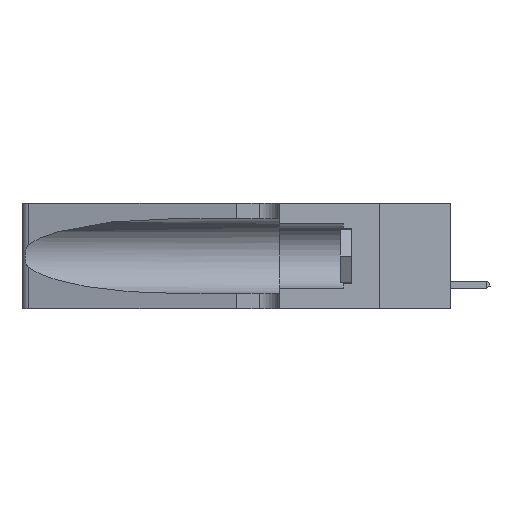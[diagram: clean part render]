
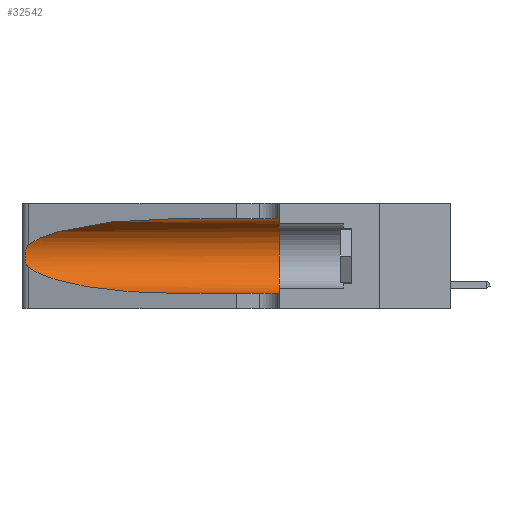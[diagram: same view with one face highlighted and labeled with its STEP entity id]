
A CAD part, left-side view. The second image highlights one B-rep face of the part: STEP entity #32542.
In plain terms, the highlighted cylindrical face has radius 3.308 mm (diameter 6.617 mm), a partial arc.
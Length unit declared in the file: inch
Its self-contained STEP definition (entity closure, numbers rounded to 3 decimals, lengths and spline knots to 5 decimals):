
#226 = CARTESIAN_POINT ( 'NONE',  ( 0.25487, 1.22718, 0.22369 ) ) ;
#278 = CIRCLE ( 'NONE', #18282, 0.13025 ) ;
#740 = ORIENTED_EDGE ( 'NONE', *, *, #19735, .T. ) ;
#765 = VERTEX_POINT ( 'NONE', #9057 ) ;
#1248 = CARTESIAN_POINT ( 'NONE',  ( 0.1305, 1.61858, 0.05475 ) ) ;
#1630 = CARTESIAN_POINT ( 'NONE',  ( 0.1305, 0.35, 0.05475 ) ) ;
#2726 = CARTESIAN_POINT ( 'NONE',  ( 0.26075, 1.23896, 0.178 ) ) ;
#3326 = CARTESIAN_POINT ( 'NONE',  ( 0.1305, 1.61858, 0.31525 ) ) ;
#3805 = ORIENTED_EDGE ( 'NONE', *, *, #20545, .T. ) ;
#3929 = B_SPLINE_CURVE_WITH_KNOTS ( 'NONE', 3,
 ( #226, #7706, #4819, #17422, #25188, #22457, #17846, #2726, #7383, #14912, #22665, #12674, #10114, #32436 ),
 .UNSPECIFIED., .F., .F.,
 ( 4, 2, 2, 2, 2, 2, 4 ),
 ( 0., 0.00027, 0.00053, 0.00107, 0.0016, 0.00187, 0.00214 ),
 .UNSPECIFIED. ) ;
#4819 = CARTESIAN_POINT ( 'NONE',  ( 0.25639, 1.23184, 0.21858 ) ) ;
#5187 = VERTEX_POINT ( 'NONE', #27787 ) ;
#6361 = CARTESIAN_POINT ( 'NONE',  ( 0.25487, 1.22718, 0.22369 ) ) ;
#7383 = CARTESIAN_POINT ( 'NONE',  ( 0.26017, 1.23833, 0.17102 ) ) ;
#7706 = CARTESIAN_POINT ( 'NONE',  ( 0.25555, 1.22994, 0.2215 ) ) ;
#7858 = DIRECTION ( 'NONE',  ( 0., -1., 0. ) ) ;
#7900 = DIRECTION ( 'NONE',  ( 0., 0., 1. ) ) ;
#7995 = AXIS2_PLACEMENT_3D ( 'NONE', #12934, #7858, #20523 ) ;
#8211 = CARTESIAN_POINT ( 'NONE',  ( 0.25487, 1.22718, 0.22369 ) ) ;
#8829 =( BOUNDED_CURVE ( )  B_SPLINE_CURVE ( 3, ( #16374, #31018, #21887, #22630 ),
 .UNSPECIFIED., .F., .T. ) 
 B_SPLINE_CURVE_WITH_KNOTS ( ( 4, 4 ),
 ( 3.44316, 4.71239 ),
 .UNSPECIFIED. ) 
 CURVE ( )  GEOMETRIC_REPRESENTATION_ITEM ( )  RATIONAL_B_SPLINE_CURVE ( ( 1., 0.87, 0.87, 1. ) ) 
 REPRESENTATION_ITEM ( '' )  );
#8934 = CARTESIAN_POINT ( 'NONE',  ( 0.2373, 1.15595, 0.28018 ) ) ;
#9057 = CARTESIAN_POINT ( 'NONE',  ( 0.1305, 0.72297, 0.31525 ) ) ;
#9798 = VECTOR ( 'NONE', #21502, 39.37008 ) ;
#10114 = CARTESIAN_POINT ( 'NONE',  ( 0.25555, 1.22993, 0.14849 ) ) ;
#11709 = VECTOR ( 'NONE', #28856, 39.37008 ) ;
#12117 = LINE ( 'NONE', #3326, #11709 ) ;
#12324 = ORIENTED_EDGE ( 'NONE', *, *, #14534, .T. ) ;
#12674 = CARTESIAN_POINT ( 'NONE',  ( 0.25639, 1.23186, 0.15144 ) ) ;
#12934 = CARTESIAN_POINT ( 'NONE',  ( 0.1305, 1.61858, 0.185 ) ) ;
#13304 = CARTESIAN_POINT ( 'NONE',  ( 0.25487, 1.22718, 0.14631 ) ) ;
#14457 = VERTEX_POINT ( 'NONE', #13304 ) ;
#14534 = EDGE_CURVE ( 'NONE', #14457, #23124, #8829, .T. ) ;
#14756 = CARTESIAN_POINT ( 'NONE',  ( 0.1305, 0.72297, 0.05475 ) ) ;
#14786 = VERTEX_POINT ( 'NONE', #6361 ) ;
#14912 = CARTESIAN_POINT ( 'NONE',  ( 0.25856, 1.23593, 0.16098 ) ) ;
#15291 = DIRECTION ( 'NONE',  ( 0., 1., 0. ) ) ;
#15694 = LINE ( 'NONE', #1248, #9798 ) ;
#16374 = CARTESIAN_POINT ( 'NONE',  ( 0.25487, 1.22718, 0.14631 ) ) ;
#17422 = CARTESIAN_POINT ( 'NONE',  ( 0.25787, 1.23484, 0.2124 ) ) ;
#17671 = CARTESIAN_POINT ( 'NONE',  ( 0.1305, 0.72297, 0.31525 ) ) ;
#17846 = CARTESIAN_POINT ( 'NONE',  ( 0.26075, 1.23896, 0.19203 ) ) ;
#18282 = AXIS2_PLACEMENT_3D ( 'NONE', #30303, #15291, #7900 ) ;
#19403 = CARTESIAN_POINT ( 'NONE',  ( 0.18966, 0.96281, 0.31525 ) ) ;
#19489 = VERTEX_POINT ( 'NONE', #1630 ) ;
#19592 = ORIENTED_EDGE ( 'NONE', *, *, #21495, .F. ) ;
#19735 = EDGE_CURVE ( 'NONE', #765, #14786, #29153, .T. ) ;
#20523 = DIRECTION ( 'NONE',  ( 0., 0., -1. ) ) ;
#20545 = EDGE_CURVE ( 'NONE', #23124, #19489, #15694, .T. ) ;
#20755 = EDGE_CURVE ( 'NONE', #14786, #14457, #3929, .T. ) ;
#21495 = EDGE_CURVE ( 'NONE', #765, #5187, #12117, .T. ) ;
#21502 = DIRECTION ( 'NONE',  ( 0., -1., 0. ) ) ;
#21887 = CARTESIAN_POINT ( 'NONE',  ( 0.18966, 0.96281, 0.05475 ) ) ;
#22457 = CARTESIAN_POINT ( 'NONE',  ( 0.26018, 1.23835, 0.19895 ) ) ;
#22547 = ORIENTED_EDGE ( 'NONE', *, *, #20755, .T. ) ;
#22630 = CARTESIAN_POINT ( 'NONE',  ( 0.1305, 0.72297, 0.05475 ) ) ;
#22665 = CARTESIAN_POINT ( 'NONE',  ( 0.25789, 1.23486, 0.15765 ) ) ;
#23124 = VERTEX_POINT ( 'NONE', #14756 ) ;
#25188 = CARTESIAN_POINT ( 'NONE',  ( 0.25854, 1.2359, 0.20912 ) ) ;
#26749 = CYLINDRICAL_SURFACE ( 'NONE', #7995, 0.13025 ) ;
#27532 = FACE_OUTER_BOUND ( 'NONE', #31613, .T. ) ;
#27787 = CARTESIAN_POINT ( 'NONE',  ( 0.1305, 0.35, 0.31525 ) ) ;
#28856 = DIRECTION ( 'NONE',  ( 0., -1., 0. ) ) ;
#29153 =( BOUNDED_CURVE ( )  B_SPLINE_CURVE ( 3, ( #17671, #19403, #8934, #8211 ),
 .UNSPECIFIED., .F., .T. ) 
 B_SPLINE_CURVE_WITH_KNOTS ( ( 4, 4 ),
 ( 1.5708, 2.84003 ),
 .UNSPECIFIED. ) 
 CURVE ( )  GEOMETRIC_REPRESENTATION_ITEM ( )  RATIONAL_B_SPLINE_CURVE ( ( 1., 0.87, 0.87, 1. ) ) 
 REPRESENTATION_ITEM ( '' )  );
#29223 = ORIENTED_EDGE ( 'NONE', *, *, #29833, .F. ) ;
#29833 = EDGE_CURVE ( 'NONE', #5187, #19489, #278, .T. ) ;
#30303 = CARTESIAN_POINT ( 'NONE',  ( 0.1305, 0.35, 0.185 ) ) ;
#31018 = CARTESIAN_POINT ( 'NONE',  ( 0.2373, 1.15595, 0.08982 ) ) ;
#31613 = EDGE_LOOP ( 'NONE', ( #740, #22547, #12324, #3805, #29223, #19592 ) ) ;
#32436 = CARTESIAN_POINT ( 'NONE',  ( 0.25487, 1.22718, 0.14631 ) ) ;
#32542 = ADVANCED_FACE ( 'NONE', ( #27532 ), #26749, .F. ) ;
